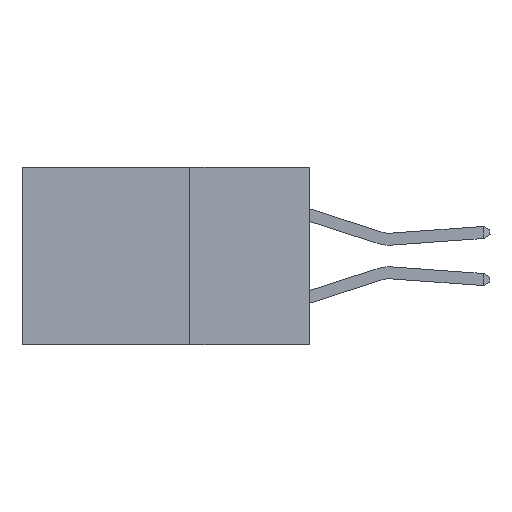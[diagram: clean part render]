
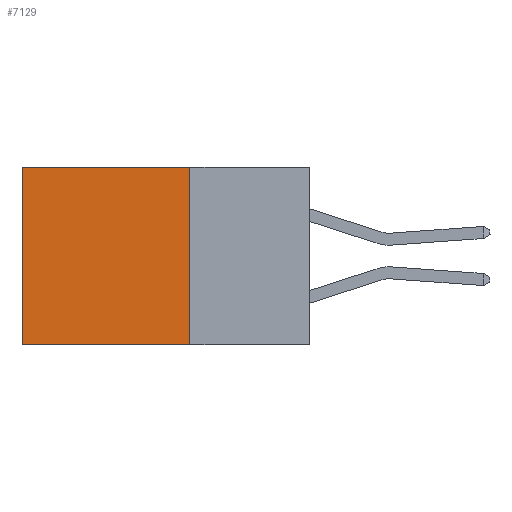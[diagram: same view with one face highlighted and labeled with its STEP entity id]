
A CAD part, left-side view. The second image highlights one B-rep face of the part: STEP entity #7129.
In plain terms, the highlighted planar face has unit normal (-1, 0, 0).
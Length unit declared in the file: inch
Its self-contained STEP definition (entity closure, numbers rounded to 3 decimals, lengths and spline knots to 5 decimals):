
#86 = LINE ( 'NONE', #3758, #264 ) ;
#172 = CARTESIAN_POINT ( 'NONE',  ( 0.2615, 0.25, -0.37 ) ) ;
#264 = VECTOR ( 'NONE', #3072, 39.37008 ) ;
#1571 = VERTEX_POINT ( 'NONE', #8045 ) ;
#1619 = DIRECTION ( 'NONE',  ( 0., 0., -1. ) ) ;
#1763 = DIRECTION ( 'NONE',  ( 0., 0., -1. ) ) ;
#1813 = VECTOR ( 'NONE', #7052, 39.37008 ) ;
#1979 = LINE ( 'NONE', #3531, #1813 ) ;
#2455 = ORIENTED_EDGE ( 'NONE', *, *, #8077, .F. ) ;
#2625 = ORIENTED_EDGE ( 'NONE', *, *, #8063, .T. ) ;
#2772 = VECTOR ( 'NONE', #1619, 39.37008 ) ;
#3072 = DIRECTION ( 'NONE',  ( 0., 1., 0. ) ) ;
#3121 = PLANE ( 'NONE',  #8518 ) ;
#3127 = VERTEX_POINT ( 'NONE', #5708 ) ;
#3531 = CARTESIAN_POINT ( 'NONE',  ( 0.2615, 0.25, -0.37 ) ) ;
#3568 = VERTEX_POINT ( 'NONE', #7647 ) ;
#3758 = CARTESIAN_POINT ( 'NONE',  ( 0.2615, 0.25, 0. ) ) ;
#4081 = CARTESIAN_POINT ( 'NONE',  ( 0.2615, 0.25, 0. ) ) ;
#4804 = ORIENTED_EDGE ( 'NONE', *, *, #6719, .F. ) ;
#5335 = LINE ( 'NONE', #6757, #2772 ) ;
#5425 = DIRECTION ( 'NONE',  ( 1., 0., 0. ) ) ;
#5708 = CARTESIAN_POINT ( 'NONE',  ( 0.2615, 0.6, -0.37 ) ) ;
#6320 = VERTEX_POINT ( 'NONE', #4081 ) ;
#6605 = EDGE_LOOP ( 'NONE', ( #8666, #4804, #2455, #2625 ) ) ;
#6628 = LINE ( 'NONE', #7433, #7802 ) ;
#6719 = EDGE_CURVE ( 'NONE', #3568, #3127, #1979, .T. ) ;
#6757 = CARTESIAN_POINT ( 'NONE',  ( 0.2615, 0.25, -0.37 ) ) ;
#7052 = DIRECTION ( 'NONE',  ( 0., 1., 0. ) ) ;
#7129 = ADVANCED_FACE ( 'NONE', ( #8987 ), #3121, .F. ) ;
#7433 = CARTESIAN_POINT ( 'NONE',  ( 0.2615, 0.6, -0.37 ) ) ;
#7647 = CARTESIAN_POINT ( 'NONE',  ( 0.2615, 0.25, -0.37 ) ) ;
#7802 = VECTOR ( 'NONE', #9584, 39.37008 ) ;
#8045 = CARTESIAN_POINT ( 'NONE',  ( 0.2615, 0.6, 0. ) ) ;
#8063 = EDGE_CURVE ( 'NONE', #6320, #1571, #86, .T. ) ;
#8077 = EDGE_CURVE ( 'NONE', #6320, #3568, #5335, .T. ) ;
#8518 = AXIS2_PLACEMENT_3D ( 'NONE', #172, #5425, #1763 ) ;
#8666 = ORIENTED_EDGE ( 'NONE', *, *, #9382, .T. ) ;
#8987 = FACE_OUTER_BOUND ( 'NONE', #6605, .T. ) ;
#9382 = EDGE_CURVE ( 'NONE', #1571, #3127, #6628, .T. ) ;
#9584 = DIRECTION ( 'NONE',  ( 0., 0., -1. ) ) ;
